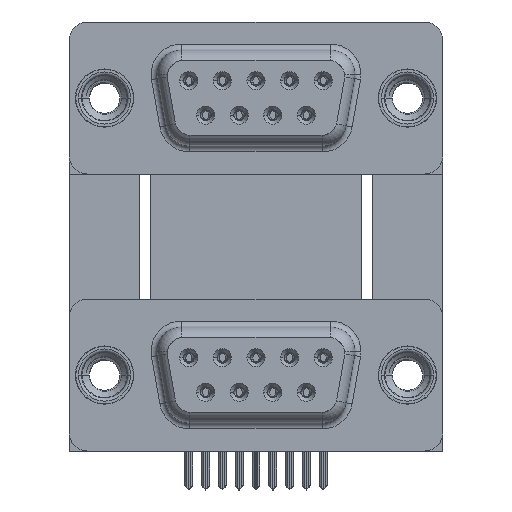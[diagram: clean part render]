
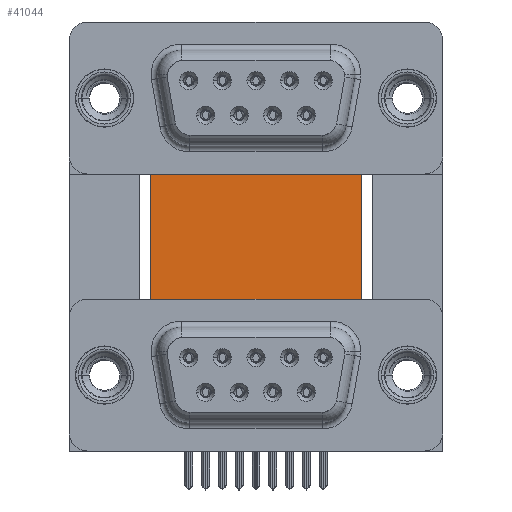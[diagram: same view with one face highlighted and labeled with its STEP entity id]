
A CAD part, top view. The second image highlights one B-rep face of the part: STEP entity #41044.
In plain terms, the highlighted planar face has unit normal (0, 0, 1).
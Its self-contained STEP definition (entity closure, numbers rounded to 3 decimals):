
#507 = EDGE_CURVE ( 'NONE', #24436, #10979, #3127, .T. ) ;
#1242 = ORIENTED_EDGE ( 'NONE', *, *, #24439, .T. ) ;
#2883 = CARTESIAN_POINT ( 'NONE',  ( 21.2, 16.585, -12. ) ) ;
#3127 = LINE ( 'NONE', #23838, #12039 ) ;
#3253 = LINE ( 'NONE', #19481, #18090 ) ;
#3899 = ORIENTED_EDGE ( 'NONE', *, *, #31200, .T. ) ;
#4303 = CARTESIAN_POINT ( 'NONE',  ( 2.9, -3.735, -12. ) ) ;
#4347 = EDGE_CURVE ( 'NONE', #10979, #42657, #20274, .T. ) ;
#4403 = CARTESIAN_POINT ( 'NONE',  ( 22.59, -4.635, -12. ) ) ;
#4863 = CARTESIAN_POINT ( 'NONE',  ( 2.4, -4.635, -12. ) ) ;
#5231 = CARTESIAN_POINT ( 'NONE',  ( 22.59, -4.635, -12. ) ) ;
#5374 = CARTESIAN_POINT ( 'NONE',  ( 21.2, 16.585, -12. ) ) ;
#5453 = DIRECTION ( 'NONE',  ( -0.336, 0.942, 0. ) ) ;
#5674 = CARTESIAN_POINT ( 'NONE',  ( 3.79, 16.585, -12. ) ) ;
#7077 = CARTESIAN_POINT ( 'NONE',  ( 2.9, -4.635, -12. ) ) ;
#7637 = VERTEX_POINT ( 'NONE', #37615 ) ;
#8741 = LINE ( 'NONE', #5374, #14217 ) ;
#10768 = LINE ( 'NONE', #26984, #28387 ) ;
#10979 = VERTEX_POINT ( 'NONE', #4303 ) ;
#11610 = PLANE ( 'NONE',  #24910 ) ;
#11829 = ORIENTED_EDGE ( 'NONE', *, *, #4347, .T. ) ;
#11910 = DIRECTION ( 'NONE',  ( 0., -1., 0. ) ) ;
#12039 = VECTOR ( 'NONE', #37575, 1000. ) ;
#12363 = CARTESIAN_POINT ( 'NONE',  ( 3.79, -0.735, -12. ) ) ;
#13304 = ORIENTED_EDGE ( 'NONE', *, *, #41356, .T. ) ;
#14217 = VECTOR ( 'NONE', #11910, 1000. ) ;
#14276 = DIRECTION ( 'NONE',  ( 1., 0., 0. ) ) ;
#14559 = DIRECTION ( 'NONE',  ( 0., 0., -1. ) ) ;
#14790 = FACE_OUTER_BOUND ( 'NONE', #16534, .T. ) ;
#15007 = CARTESIAN_POINT ( 'NONE',  ( 2.9, -4.635, -12. ) ) ;
#16534 = EDGE_LOOP ( 'NONE', ( #11829, #34053, #3899, #36462, #27087, #23959, #38827, #1242, #13304, #36574 ) ) ;
#16719 = CARTESIAN_POINT ( 'NONE',  ( 22.09, -3.735, -12. ) ) ;
#18090 = VECTOR ( 'NONE', #30717, 1000. ) ;
#19188 = EDGE_CURVE ( 'NONE', #31585, #39796, #32239, .T. ) ;
#19268 = VECTOR ( 'NONE', #40302, 1000. ) ;
#19481 = CARTESIAN_POINT ( 'NONE',  ( 22.09, -3.735, -12. ) ) ;
#19833 = CARTESIAN_POINT ( 'NONE',  ( 3.79, -3.735, -12. ) ) ;
#20065 = LINE ( 'NONE', #5674, #23871 ) ;
#20274 = LINE ( 'NONE', #19833, #19268 ) ;
#21799 = CARTESIAN_POINT ( 'NONE',  ( 3.79, 16.585, -12. ) ) ;
#21948 = LINE ( 'NONE', #4863, #39731 ) ;
#22026 = LINE ( 'NONE', #21799, #38286 ) ;
#22826 = VERTEX_POINT ( 'NONE', #12363 ) ;
#23601 = EDGE_CURVE ( 'NONE', #7637, #22826, #20065, .T. ) ;
#23838 = CARTESIAN_POINT ( 'NONE',  ( 2.9, -3.735, -12. ) ) ;
#23871 = VECTOR ( 'NONE', #32918, 1000. ) ;
#23959 = ORIENTED_EDGE ( 'NONE', *, *, #27746, .F. ) ;
#24414 = CARTESIAN_POINT ( 'NONE',  ( 22.09, -4.635, -12. ) ) ;
#24436 = VERTEX_POINT ( 'NONE', #15007 ) ;
#24439 = EDGE_CURVE ( 'NONE', #22826, #43287, #21948, .T. ) ;
#24910 = AXIS2_PLACEMENT_3D ( 'NONE', #28484, #14559, #42215 ) ;
#25102 = VECTOR ( 'NONE', #5453, 1000. ) ;
#25849 = EDGE_CURVE ( 'NONE', #42657, #26880, #3253, .T. ) ;
#26880 = VERTEX_POINT ( 'NONE', #24414 ) ;
#26984 = CARTESIAN_POINT ( 'NONE',  ( 22.09, -4.635, -12. ) ) ;
#27087 = ORIENTED_EDGE ( 'NONE', *, *, #43154, .F. ) ;
#27563 = CARTESIAN_POINT ( 'NONE',  ( 2.4, -4.635, -12. ) ) ;
#27746 = EDGE_CURVE ( 'NONE', #7637, #39646, #22026, .T. ) ;
#28208 = LINE ( 'NONE', #7077, #44367 ) ;
#28387 = VECTOR ( 'NONE', #40712, 1000. ) ;
#28484 = CARTESIAN_POINT ( 'NONE',  ( 3.79, 16.585, -12. ) ) ;
#28516 = CARTESIAN_POINT ( 'NONE',  ( 21.2, -0.735, -12. ) ) ;
#28708 = DIRECTION ( 'NONE',  ( -0.336, -0.942, 0. ) ) ;
#30717 = DIRECTION ( 'NONE',  ( 0., -1., 0. ) ) ;
#31200 = EDGE_CURVE ( 'NONE', #26880, #31585, #10768, .T. ) ;
#31585 = VERTEX_POINT ( 'NONE', #4403 ) ;
#32239 = LINE ( 'NONE', #5231, #25102 ) ;
#32918 = DIRECTION ( 'NONE',  ( 0., -1., 0. ) ) ;
#34053 = ORIENTED_EDGE ( 'NONE', *, *, #25849, .T. ) ;
#35321 = DIRECTION ( 'NONE',  ( 1., 0., 0. ) ) ;
#36462 = ORIENTED_EDGE ( 'NONE', *, *, #19188, .T. ) ;
#36574 = ORIENTED_EDGE ( 'NONE', *, *, #507, .T. ) ;
#37575 = DIRECTION ( 'NONE',  ( 0., 1., 0. ) ) ;
#37615 = CARTESIAN_POINT ( 'NONE',  ( 3.79, 16.585, -12. ) ) ;
#38286 = VECTOR ( 'NONE', #35321, 1000. ) ;
#38827 = ORIENTED_EDGE ( 'NONE', *, *, #23601, .T. ) ;
#39646 = VERTEX_POINT ( 'NONE', #2883 ) ;
#39731 = VECTOR ( 'NONE', #28708, 1000. ) ;
#39796 = VERTEX_POINT ( 'NONE', #28516 ) ;
#40302 = DIRECTION ( 'NONE',  ( 1., 0., 0. ) ) ;
#40712 = DIRECTION ( 'NONE',  ( 1., 0., 0. ) ) ;
#41044 = ADVANCED_FACE ( 'NONE', ( #14790 ), #11610, .F. ) ;
#41356 = EDGE_CURVE ( 'NONE', #43287, #24436, #28208, .T. ) ;
#42215 = DIRECTION ( 'NONE',  ( -1., 0., 0. ) ) ;
#42657 = VERTEX_POINT ( 'NONE', #16719 ) ;
#43154 = EDGE_CURVE ( 'NONE', #39646, #39796, #8741, .T. ) ;
#43287 = VERTEX_POINT ( 'NONE', #27563 ) ;
#44367 = VECTOR ( 'NONE', #14276, 1000. ) ;
